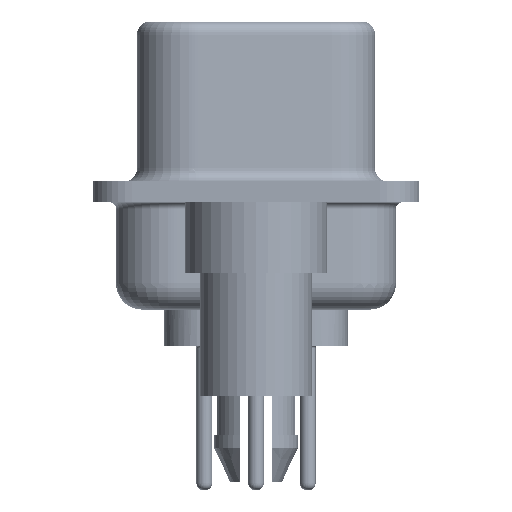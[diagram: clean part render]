
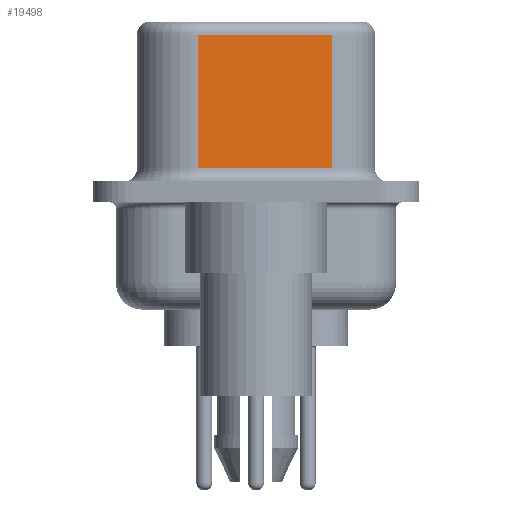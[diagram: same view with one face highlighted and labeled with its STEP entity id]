
A CAD part, left-side view. The second image highlights one B-rep face of the part: STEP entity #19498.
In plain terms, the highlighted planar face has unit normal (-0.985, -0.174, 0).
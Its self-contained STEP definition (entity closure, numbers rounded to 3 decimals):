
#98 = VERTEX_POINT ( 'NONE', #28422 ) ;
#234 = CARTESIAN_POINT ( 'NONE',  ( 3.68, 2.203, 6.52 ) ) ;
#788 = VECTOR ( 'NONE', #5701, 1000. ) ;
#1601 = LINE ( 'NONE', #29032, #788 ) ;
#2959 = VERTEX_POINT ( 'NONE', #32162 ) ;
#4635 = EDGE_CURVE ( 'NONE', #2959, #4946, #9915, .T. ) ;
#4946 = VERTEX_POINT ( 'NONE', #24078 ) ;
#5056 = PLANE ( 'NONE',  #31564 ) ;
#5701 = DIRECTION ( 'NONE',  ( 0.174, -0.985, 0. ) ) ;
#5943 = CARTESIAN_POINT ( 'NONE',  ( 3.68, 2.203, 0.9 ) ) ;
#6100 = FACE_OUTER_BOUND ( 'NONE', #16851, .T. ) ;
#9915 = LINE ( 'NONE', #18677, #22905 ) ;
#10320 = DIRECTION ( 'NONE',  ( -0.174, 0.985, 0. ) ) ;
#10724 = VECTOR ( 'NONE', #17148, 1000. ) ;
#14081 = LINE ( 'NONE', #234, #21003 ) ;
#14519 = CARTESIAN_POINT ( 'NONE',  ( 4.58, -2.897, 6.52 ) ) ;
#16838 = DIRECTION ( 'NONE',  ( -0.174, 0.985, 0. ) ) ;
#16851 = EDGE_LOOP ( 'NONE', ( #18933, #30185, #26006, #31203 ) ) ;
#17148 = DIRECTION ( 'NONE',  ( 0., 0., -1. ) ) ;
#17433 = EDGE_CURVE ( 'NONE', #2959, #98, #31229, .T. ) ;
#17877 = VERTEX_POINT ( 'NONE', #5943 ) ;
#18677 = CARTESIAN_POINT ( 'NONE',  ( 4.58, -2.897, 6.02 ) ) ;
#18933 = ORIENTED_EDGE ( 'NONE', *, *, #17433, .F. ) ;
#19498 = ADVANCED_FACE ( 'NONE', ( #6100 ), #5056, .F. ) ;
#21003 = VECTOR ( 'NONE', #21044, 1000. ) ;
#21044 = DIRECTION ( 'NONE',  ( 0., 0., -1. ) ) ;
#22905 = VECTOR ( 'NONE', #16838, 1000. ) ;
#23252 = CARTESIAN_POINT ( 'NONE',  ( 4.58, -2.897, 6.52 ) ) ;
#24078 = CARTESIAN_POINT ( 'NONE',  ( 3.68, 2.203, 6.02 ) ) ;
#25644 = EDGE_CURVE ( 'NONE', #17877, #98, #1601, .T. ) ;
#25844 = DIRECTION ( 'NONE',  ( 0.985, 0.174, 0. ) ) ;
#26006 = ORIENTED_EDGE ( 'NONE', *, *, #30803, .T. ) ;
#28422 = CARTESIAN_POINT ( 'NONE',  ( 4.58, -2.897, 0.9 ) ) ;
#29032 = CARTESIAN_POINT ( 'NONE',  ( 4.58, -2.897, 0.9 ) ) ;
#30185 = ORIENTED_EDGE ( 'NONE', *, *, #4635, .T. ) ;
#30803 = EDGE_CURVE ( 'NONE', #4946, #17877, #14081, .T. ) ;
#31203 = ORIENTED_EDGE ( 'NONE', *, *, #25644, .T. ) ;
#31229 = LINE ( 'NONE', #14519, #10724 ) ;
#31564 = AXIS2_PLACEMENT_3D ( 'NONE', #23252, #25844, #10320 ) ;
#32162 = CARTESIAN_POINT ( 'NONE',  ( 4.58, -2.897, 6.02 ) ) ;
